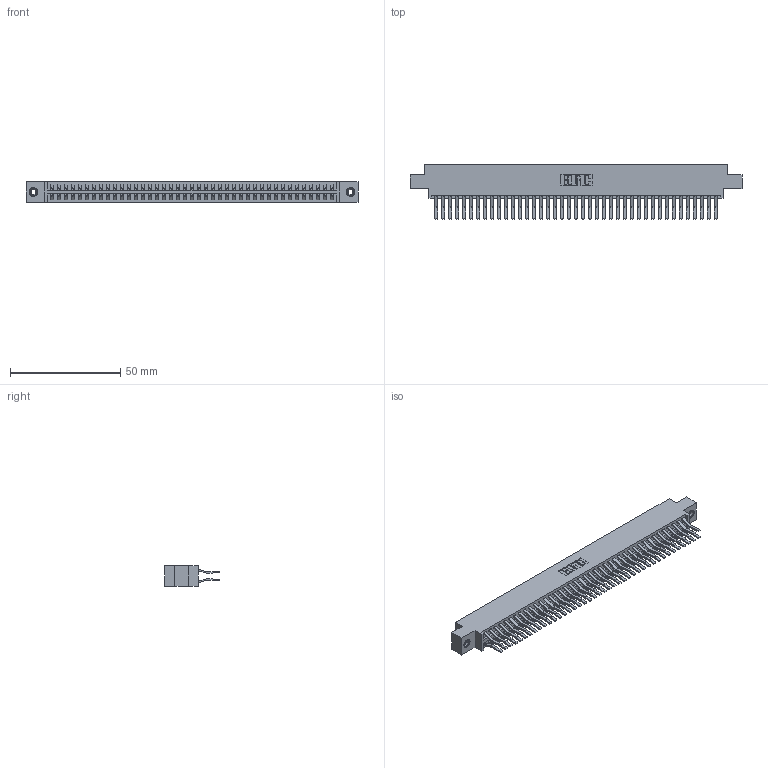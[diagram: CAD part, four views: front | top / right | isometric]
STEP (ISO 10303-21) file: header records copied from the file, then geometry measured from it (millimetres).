
FILE_DESCRIPTION (( 'STEP AP203' ), '1' );
FILE_NAME ('396-082-560-808.STEP', '2018-09-10T00:10:53', ( '' ), ( '' ), 'SwSTEP 2.0', 'SolidWorks 2016', '' );
FILE_SCHEMA (( 'CONFIG_CONTROL_DESIGN' ));
Length unit declared in the file: inch
Products named in the file (4): 345-292-001_560 Tail; 345-250-001_345-250-003-102; 396-082-560-808; 346 Part_0.170 Offset - 0.156 Dia-TI
Assembly tree (85 placements, depth 2):
  396-082-560-808
    346 Part_0.170 Offset - 0.156 Dia-TI
    345-292-001_560 Tail  x82
    345-250-001_345-250-003-102  x2
Bounding box: 150.75 x 24.78 x 9.4 mm (x, y, z)
Volume: 15068.5 mm3; surface area: 22330.5 mm2
Topology: 85 solids, 85 shells, 4614 faces, 13679 edges, 9002 vertices
Faces by surface type: plane 2982, cylinder 1616, cone 12, torus 4
Entity records: 28298 total; most frequent: CARTESIAN_POINT 4651, ORIENTED_EDGE 4578, DIRECTION 4179, EDGE_CURVE 2289, LINE 1969, VECTOR 1969, VERTEX_POINT 1520, AXIS2_PLACEMENT_3D 1105
